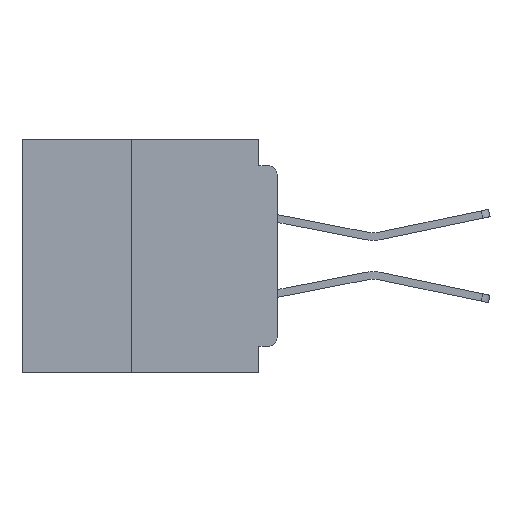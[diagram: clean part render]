
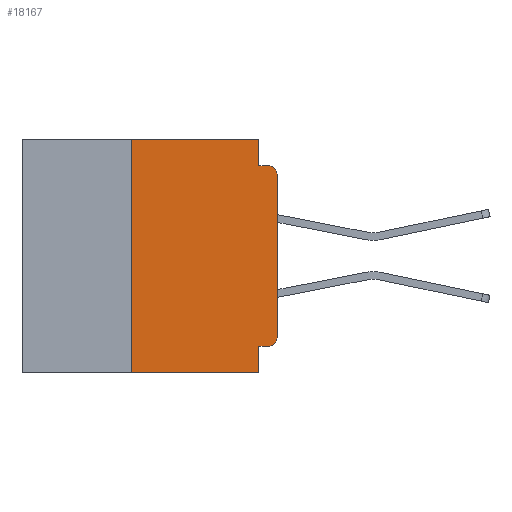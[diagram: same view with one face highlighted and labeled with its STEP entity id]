
A CAD part, left-side view. The second image highlights one B-rep face of the part: STEP entity #18167.
In plain terms, the highlighted planar face has unit normal (-1, 0, 0).
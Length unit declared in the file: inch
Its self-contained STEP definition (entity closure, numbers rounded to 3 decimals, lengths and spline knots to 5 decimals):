
#739 = PLANE ( 'NONE',  #33730 ) ;
#1636 = LINE ( 'NONE', #19019, #10116 ) ;
#1706 = VERTEX_POINT ( 'NONE', #13372 ) ;
#2199 = LINE ( 'NONE', #10047, #39440 ) ;
#5244 = DIRECTION ( 'NONE',  ( 0., -1., 0. ) ) ;
#5285 = VERTEX_POINT ( 'NONE', #39682 ) ;
#6077 = AXIS2_PLACEMENT_3D ( 'NONE', #31866, #10290, #35509 ) ;
#6089 = EDGE_CURVE ( 'NONE', #19567, #6594, #25325, .T. ) ;
#6140 = VECTOR ( 'NONE', #26520, 39.37008 ) ;
#6402 = VECTOR ( 'NONE', #14477, 39.37008 ) ;
#6594 = VERTEX_POINT ( 'NONE', #32925 ) ;
#6983 = EDGE_CURVE ( 'NONE', #6594, #25409, #7831, .T. ) ;
#7440 = AXIS2_PLACEMENT_3D ( 'NONE', #17106, #42334, #20763 ) ;
#7831 = CIRCLE ( 'NONE', #7440, 0.015 ) ;
#8056 = DIRECTION ( 'NONE',  ( 0., 0., -1. ) ) ;
#8774 = ORIENTED_EDGE ( 'NONE', *, *, #38095, .T. ) ;
#9898 = LINE ( 'NONE', #29269, #35274 ) ;
#10047 = CARTESIAN_POINT ( 'NONE',  ( 0., 0., -0.045 ) ) ;
#10116 = VECTOR ( 'NONE', #37011, 39.37008 ) ;
#10290 = DIRECTION ( 'NONE',  ( -1., 0., 0. ) ) ;
#10293 = LINE ( 'NONE', #17302, #28332 ) ;
#10648 = ORIENTED_EDGE ( 'NONE', *, *, #40503, .F. ) ;
#11836 = EDGE_CURVE ( 'NONE', #29509, #45529, #13431, .T. ) ;
#12144 = ORIENTED_EDGE ( 'NONE', *, *, #6983, .T. ) ;
#13372 = CARTESIAN_POINT ( 'NONE',  ( 0., 0.25, -0.4 ) ) ;
#13431 = LINE ( 'NONE', #39367, #21922 ) ;
#13662 = DIRECTION ( 'NONE',  ( 0., -1., 0. ) ) ;
#13983 = VERTEX_POINT ( 'NONE', #27628 ) ;
#14477 = DIRECTION ( 'NONE',  ( 0., 0., -1. ) ) ;
#15626 = CARTESIAN_POINT ( 'NONE',  ( 0., 0., 0. ) ) ;
#15762 = LINE ( 'NONE', #37713, #33806 ) ;
#15981 = LINE ( 'NONE', #17946, #6402 ) ;
#17106 = CARTESIAN_POINT ( 'NONE',  ( 0., 0.015, -0.06 ) ) ;
#17302 = CARTESIAN_POINT ( 'NONE',  ( 0., 0.25, -0.4 ) ) ;
#17946 = CARTESIAN_POINT ( 'NONE',  ( 0., 0.031, -0.4 ) ) ;
#18167 = ADVANCED_FACE ( 'NONE', ( #37486 ), #739, .F. ) ;
#18204 = CARTESIAN_POINT ( 'NONE',  ( 0., 0.015, -0.045 ) ) ;
#19019 = CARTESIAN_POINT ( 'NONE',  ( 0., 0.031, 0. ) ) ;
#19567 = VERTEX_POINT ( 'NONE', #28263 ) ;
#20651 = ORIENTED_EDGE ( 'NONE', *, *, #36014, .F. ) ;
#20763 = DIRECTION ( 'NONE',  ( 0., 0., -1. ) ) ;
#21393 = DIRECTION ( 'NONE',  ( 0., 1., 0. ) ) ;
#21922 = VECTOR ( 'NONE', #21393, 39.37008 ) ;
#24124 = ORIENTED_EDGE ( 'NONE', *, *, #11836, .F. ) ;
#25325 = LINE ( 'NONE', #15626, #6140 ) ;
#25409 = VERTEX_POINT ( 'NONE', #18204 ) ;
#25579 = ORIENTED_EDGE ( 'NONE', *, *, #6089, .T. ) ;
#26029 = CARTESIAN_POINT ( 'NONE',  ( 0., 0.437, 0. ) ) ;
#26422 = CARTESIAN_POINT ( 'NONE',  ( 0., 0.031, -0.4 ) ) ;
#26520 = DIRECTION ( 'NONE',  ( 0., 0., 1. ) ) ;
#26591 = ORIENTED_EDGE ( 'NONE', *, *, #42864, .F. ) ;
#26899 = VERTEX_POINT ( 'NONE', #27526 ) ;
#26959 = ORIENTED_EDGE ( 'NONE', *, *, #41712, .T. ) ;
#27526 = CARTESIAN_POINT ( 'NONE',  ( 0., 0.25, 0. ) ) ;
#27628 = CARTESIAN_POINT ( 'NONE',  ( 0., 0.031, -0.045 ) ) ;
#28263 = CARTESIAN_POINT ( 'NONE',  ( 0., 0., -0.34 ) ) ;
#28332 = VECTOR ( 'NONE', #35286, 39.37008 ) ;
#28394 = EDGE_CURVE ( 'NONE', #45529, #42911, #15981, .T. ) ;
#29269 = CARTESIAN_POINT ( 'NONE',  ( 0., 0.437, -0.4 ) ) ;
#29509 = VERTEX_POINT ( 'NONE', #38690 ) ;
#29634 = DIRECTION ( 'NONE',  ( 1., 0., 0. ) ) ;
#30710 = EDGE_LOOP ( 'NONE', ( #25579, #12144, #20651, #26591, #42156, #10648, #8774, #37059, #24124, #26959 ) ) ;
#31866 = CARTESIAN_POINT ( 'NONE',  ( 0., 0.015, -0.34 ) ) ;
#32890 = DIRECTION ( 'NONE',  ( 0., -1., 0. ) ) ;
#32925 = CARTESIAN_POINT ( 'NONE',  ( 0., 0., -0.06 ) ) ;
#33730 = AXIS2_PLACEMENT_3D ( 'NONE', #26029, #29634, #8056 ) ;
#33806 = VECTOR ( 'NONE', #5244, 39.37008 ) ;
#35274 = VECTOR ( 'NONE', #32890, 39.37008 ) ;
#35286 = DIRECTION ( 'NONE',  ( 0., 0., 1. ) ) ;
#35509 = DIRECTION ( 'NONE',  ( 0., 0., -1. ) ) ;
#36014 = EDGE_CURVE ( 'NONE', #13983, #25409, #2199, .T. ) ;
#37011 = DIRECTION ( 'NONE',  ( 0., 0., -1. ) ) ;
#37059 = ORIENTED_EDGE ( 'NONE', *, *, #28394, .F. ) ;
#37486 = FACE_OUTER_BOUND ( 'NONE', #30710, .T. ) ;
#37713 = CARTESIAN_POINT ( 'NONE',  ( 0., 0.437, 0. ) ) ;
#38095 = EDGE_CURVE ( 'NONE', #1706, #42911, #9898, .T. ) ;
#38638 = CARTESIAN_POINT ( 'NONE',  ( 0., 0.031, -0.355 ) ) ;
#38690 = CARTESIAN_POINT ( 'NONE',  ( 0., 0.015, -0.355 ) ) ;
#39367 = CARTESIAN_POINT ( 'NONE',  ( 0., 0., -0.355 ) ) ;
#39440 = VECTOR ( 'NONE', #13662, 39.37008 ) ;
#39682 = CARTESIAN_POINT ( 'NONE',  ( 0., 0.031, 0. ) ) ;
#40503 = EDGE_CURVE ( 'NONE', #1706, #26899, #10293, .T. ) ;
#41712 = EDGE_CURVE ( 'NONE', #29509, #19567, #43405, .T. ) ;
#42117 = EDGE_CURVE ( 'NONE', #26899, #5285, #15762, .T. ) ;
#42156 = ORIENTED_EDGE ( 'NONE', *, *, #42117, .F. ) ;
#42334 = DIRECTION ( 'NONE',  ( -1., 0., 0. ) ) ;
#42864 = EDGE_CURVE ( 'NONE', #5285, #13983, #1636, .T. ) ;
#42911 = VERTEX_POINT ( 'NONE', #26422 ) ;
#43405 = CIRCLE ( 'NONE', #6077, 0.015 ) ;
#45529 = VERTEX_POINT ( 'NONE', #38638 ) ;
